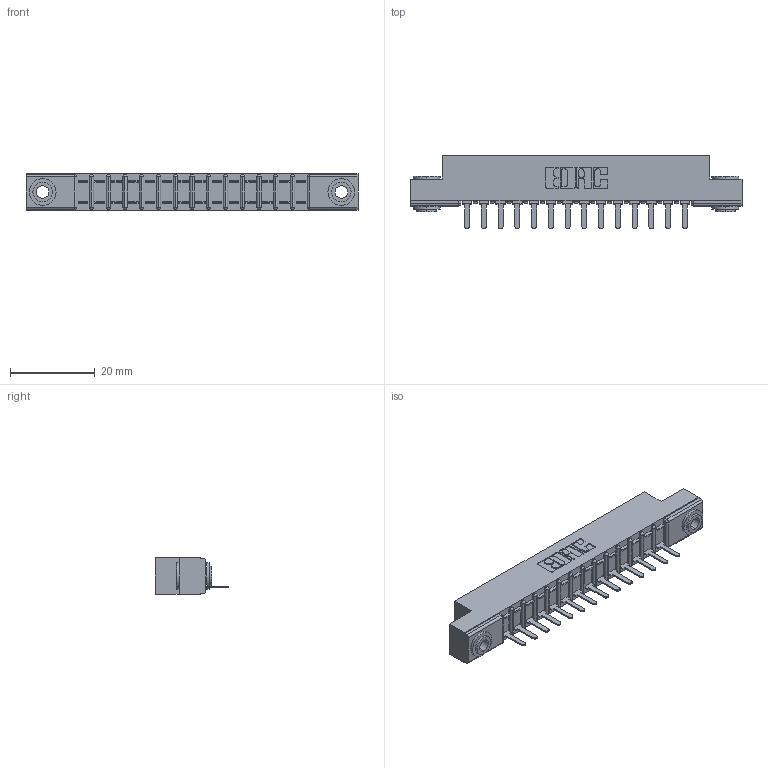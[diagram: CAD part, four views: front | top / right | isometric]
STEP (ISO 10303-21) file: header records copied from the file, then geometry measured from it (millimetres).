
FILE_DESCRIPTION (( 'STEP AP203' ), '1' );
FILE_NAME ('307-014-421-103.STEP', '2020-09-25T15:39:53', ( '' ), ( '' ), 'SwSTEP 2.0', 'SolidWorks 2020', '' );
FILE_SCHEMA (( 'CONFIG_CONTROL_DESIGN' ));
Length unit declared in the file: inch
Products named in the file (9): 307-290-002_521; 307 Part_.156 Dia Mounting Holes; 307-014-421-103; 345-250-002_345-250-002-102; 307 Part_No Mounting Lugs; 307-290-001_522; 307-014-422-201; #35205; #35858
Assembly tree (75 placements, depth 2):
  307-014-421-103
    307 Part_.156 Dia Mounting Holes
    307-290-002_521  x14
    345-250-002_345-250-002-102  x2
  307-014-422-201
    307 Part_No Mounting Lugs
    307-290-001_522  x14
Bounding box: 78.49 x 17.42 x 8.71 mm (x, y, z)
Volume: 5179.4 mm3; surface area: 9228 mm2
Topology: 17 solids, 17 shells, 1221 faces, 3683 edges, 2410 vertices
Faces by surface type: plane 724, cylinder 459, sphere 30, cone 8
Entity records: 35297 total; most frequent: CARTESIAN_POINT 5860, ORIENTED_EDGE 5798, DIRECTION 5762, EDGE_CURVE 2918, VECTOR 2202, LINE 2187, VERTEX_POINT 1911, AXIS2_PLACEMENT_3D 1772
